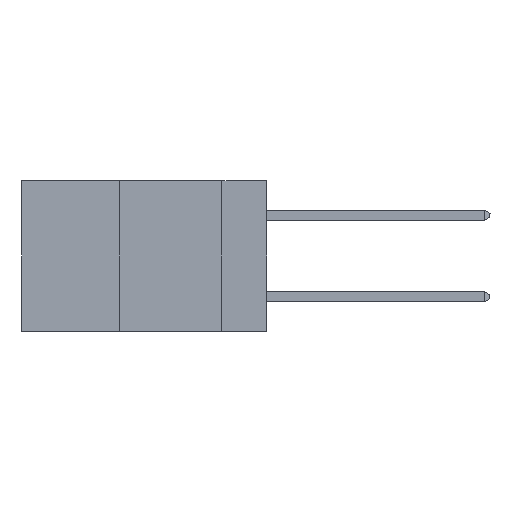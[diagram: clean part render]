
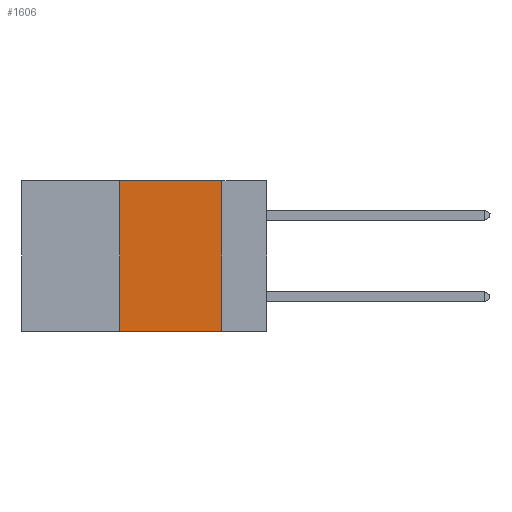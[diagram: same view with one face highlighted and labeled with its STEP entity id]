
A CAD part, left-side view. The second image highlights one B-rep face of the part: STEP entity #1606.
In plain terms, the highlighted planar face has unit normal (-1, 0, 0).
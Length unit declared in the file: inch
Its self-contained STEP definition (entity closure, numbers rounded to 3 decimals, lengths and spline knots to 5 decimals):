
#377 = CARTESIAN_POINT ( 'NONE',  ( 0., 0.6, -0.37 ) ) ;
#1528 = CARTESIAN_POINT ( 'NONE',  ( 0., 0.6, 0. ) ) ;
#1606 = ADVANCED_FACE ( 'NONE', ( #27557 ), #22283, .F. ) ;
#2939 = EDGE_CURVE ( 'NONE', #31355, #25822, #6281, .T. ) ;
#3154 = DIRECTION ( 'NONE',  ( 0., 0., -1. ) ) ;
#3168 = AXIS2_PLACEMENT_3D ( 'NONE', #30411, #4584, #3154 ) ;
#4584 = DIRECTION ( 'NONE',  ( 1., 0., 0. ) ) ;
#6281 = LINE ( 'NONE', #20666, #19618 ) ;
#7029 = CARTESIAN_POINT ( 'NONE',  ( 0., 0.36, -0.37 ) ) ;
#8322 = ORIENTED_EDGE ( 'NONE', *, *, #2939, .F. ) ;
#9500 = CARTESIAN_POINT ( 'NONE',  ( 0., 0.11, -0.37 ) ) ;
#9533 = DIRECTION ( 'NONE',  ( 0., -1., 0. ) ) ;
#9842 = VECTOR ( 'NONE', #25717, 39.37008 ) ;
#12425 = LINE ( 'NONE', #1528, #21225 ) ;
#13590 = DIRECTION ( 'NONE',  ( 0., -1., 0. ) ) ;
#13745 = DIRECTION ( 'NONE',  ( 0., 0., -1. ) ) ;
#14544 = VERTEX_POINT ( 'NONE', #7029 ) ;
#14811 = LINE ( 'NONE', #22941, #9842 ) ;
#16184 = ORIENTED_EDGE ( 'NONE', *, *, #19375, .F. ) ;
#17767 = EDGE_LOOP ( 'NONE', ( #8322, #16184, #28639, #29187 ) ) ;
#18560 = EDGE_CURVE ( 'NONE', #14544, #25822, #25009, .T. ) ;
#19375 = EDGE_CURVE ( 'NONE', #27848, #31355, #12425, .T. ) ;
#19618 = VECTOR ( 'NONE', #13745, 39.37008 ) ;
#20666 = CARTESIAN_POINT ( 'NONE',  ( 0., 0.11, 0. ) ) ;
#21225 = VECTOR ( 'NONE', #9533, 39.37008 ) ;
#22283 = PLANE ( 'NONE',  #3168 ) ;
#22941 = CARTESIAN_POINT ( 'NONE',  ( 0., 0.36, 0. ) ) ;
#25009 = LINE ( 'NONE', #377, #26241 ) ;
#25717 = DIRECTION ( 'NONE',  ( 0., 0., 1. ) ) ;
#25822 = VERTEX_POINT ( 'NONE', #9500 ) ;
#26241 = VECTOR ( 'NONE', #13590, 39.37008 ) ;
#27557 = FACE_OUTER_BOUND ( 'NONE', #17767, .T. ) ;
#27848 = VERTEX_POINT ( 'NONE', #29127 ) ;
#27857 = CARTESIAN_POINT ( 'NONE',  ( 0., 0.11, 0. ) ) ;
#28639 = ORIENTED_EDGE ( 'NONE', *, *, #30355, .F. ) ;
#29127 = CARTESIAN_POINT ( 'NONE',  ( 0., 0.36, 0. ) ) ;
#29187 = ORIENTED_EDGE ( 'NONE', *, *, #18560, .T. ) ;
#30355 = EDGE_CURVE ( 'NONE', #14544, #27848, #14811, .T. ) ;
#30411 = CARTESIAN_POINT ( 'NONE',  ( 0., 0.6, 0. ) ) ;
#31355 = VERTEX_POINT ( 'NONE', #27857 ) ;
